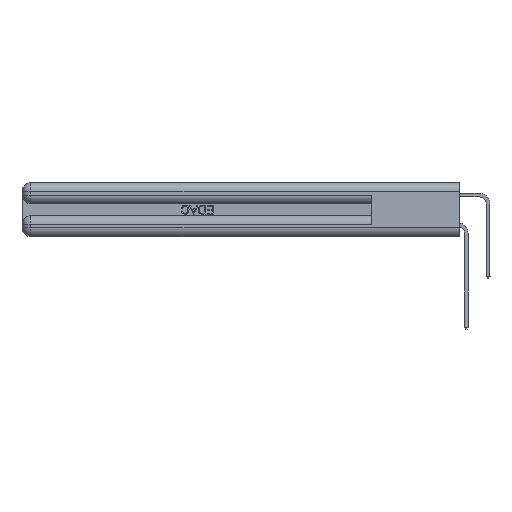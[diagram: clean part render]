
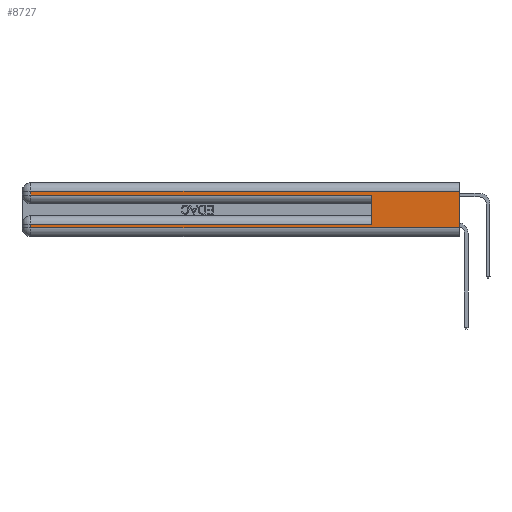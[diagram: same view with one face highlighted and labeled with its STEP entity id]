
A CAD part, left-side view. The second image highlights one B-rep face of the part: STEP entity #8727.
In plain terms, the highlighted planar face has unit normal (-1, 0, 0).
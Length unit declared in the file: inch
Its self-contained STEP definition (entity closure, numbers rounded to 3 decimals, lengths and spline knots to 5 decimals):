
#1024 = DIRECTION ( 'NONE',  ( 0., 0., -1. ) ) ;
#1883 = CARTESIAN_POINT ( 'NONE',  ( 0., 0., 0.31 ) ) ;
#2328 = EDGE_CURVE ( 'NONE', #23954, #23250, #42568, .T. ) ;
#2479 = EDGE_CURVE ( 'NONE', #31817, #32870, #14294, .T. ) ;
#4145 = VECTOR ( 'NONE', #5722, 39.37008 ) ;
#5465 = CARTESIAN_POINT ( 'NONE',  ( 0., 2.94, 0.31 ) ) ;
#5722 = DIRECTION ( 'NONE',  ( 0., 1., 0. ) ) ;
#5833 = VECTOR ( 'NONE', #11983, 39.37008 ) ;
#6729 = FACE_OUTER_BOUND ( 'NONE', #42413, .T. ) ;
#7518 = DIRECTION ( 'NONE',  ( 1., 0., 0. ) ) ;
#8128 = CARTESIAN_POINT ( 'NONE',  ( 0., 0.6, 0.145 ) ) ;
#8727 = ADVANCED_FACE ( 'NONE', ( #6729 ), #48818, .F. ) ;
#9153 = VERTEX_POINT ( 'NONE', #28420 ) ;
#10194 = VECTOR ( 'NONE', #19984, 39.37008 ) ;
#11245 = ORIENTED_EDGE ( 'NONE', *, *, #30647, .F. ) ;
#11983 = DIRECTION ( 'NONE',  ( 0., 0., 1. ) ) ;
#12028 = LINE ( 'NONE', #35225, #20831 ) ;
#12609 = DIRECTION ( 'NONE',  ( 0., -1., 0. ) ) ;
#14294 = LINE ( 'NONE', #1883, #4145 ) ;
#14537 = VECTOR ( 'NONE', #21253, 39.37008 ) ;
#14733 = CARTESIAN_POINT ( 'NONE',  ( 0., 0., 0.31 ) ) ;
#15948 = LINE ( 'NONE', #8128, #5833 ) ;
#17094 = CARTESIAN_POINT ( 'NONE',  ( 0., 0., 0.37 ) ) ;
#17153 = DIRECTION ( 'NONE',  ( 0., -1., 0. ) ) ;
#19131 = EDGE_CURVE ( 'NONE', #32870, #9153, #38466, .T. ) ;
#19954 = CARTESIAN_POINT ( 'NONE',  ( 0., 2.94, 0.37 ) ) ;
#19984 = DIRECTION ( 'NONE',  ( 0., 0., -1. ) ) ;
#20187 = CARTESIAN_POINT ( 'NONE',  ( 0., 0.6, 0.085 ) ) ;
#20487 = EDGE_CURVE ( 'NONE', #31817, #32474, #20671, .T. ) ;
#20541 = VERTEX_POINT ( 'NONE', #39964 ) ;
#20671 = LINE ( 'NONE', #17094, #29493 ) ;
#20831 = VECTOR ( 'NONE', #17153, 39.37008 ) ;
#21253 = DIRECTION ( 'NONE',  ( 0., 1., 0. ) ) ;
#21902 = ORIENTED_EDGE ( 'NONE', *, *, #34975, .T. ) ;
#23250 = VERTEX_POINT ( 'NONE', #28031 ) ;
#23479 = ORIENTED_EDGE ( 'NONE', *, *, #2328, .T. ) ;
#23733 = CARTESIAN_POINT ( 'NONE',  ( 0., 2.94, 0.37 ) ) ;
#23936 = ORIENTED_EDGE ( 'NONE', *, *, #34116, .T. ) ;
#23954 = VERTEX_POINT ( 'NONE', #28127 ) ;
#25112 = AXIS2_PLACEMENT_3D ( 'NONE', #33711, #7518, #33880 ) ;
#27268 = VECTOR ( 'NONE', #1024, 39.37008 ) ;
#27576 = CARTESIAN_POINT ( 'NONE',  ( 0., 0., 0.285 ) ) ;
#28031 = CARTESIAN_POINT ( 'NONE',  ( 0., 2.94, 0.06 ) ) ;
#28127 = CARTESIAN_POINT ( 'NONE',  ( 0., 2.94, 0.085 ) ) ;
#28420 = CARTESIAN_POINT ( 'NONE',  ( 0., 2.94, 0.285 ) ) ;
#29493 = VECTOR ( 'NONE', #47150, 39.37008 ) ;
#29786 = CARTESIAN_POINT ( 'NONE',  ( 0., 0., 0.06 ) ) ;
#30647 = EDGE_CURVE ( 'NONE', #44371, #20541, #15948, .T. ) ;
#31817 = VERTEX_POINT ( 'NONE', #14733 ) ;
#31900 = VECTOR ( 'NONE', #12609, 39.37008 ) ;
#32179 = ORIENTED_EDGE ( 'NONE', *, *, #41470, .T. ) ;
#32420 = CARTESIAN_POINT ( 'NONE',  ( 0., 0., 0.085 ) ) ;
#32474 = VERTEX_POINT ( 'NONE', #29786 ) ;
#32558 = ORIENTED_EDGE ( 'NONE', *, *, #2479, .T. ) ;
#32870 = VERTEX_POINT ( 'NONE', #5465 ) ;
#33711 = CARTESIAN_POINT ( 'NONE',  ( 0., 0., 0.37 ) ) ;
#33880 = DIRECTION ( 'NONE',  ( 0., 0., -1. ) ) ;
#34116 = EDGE_CURVE ( 'NONE', #23250, #32474, #12028, .T. ) ;
#34703 = ORIENTED_EDGE ( 'NONE', *, *, #19131, .T. ) ;
#34975 = EDGE_CURVE ( 'NONE', #9153, #20541, #35450, .T. ) ;
#34987 = ORIENTED_EDGE ( 'NONE', *, *, #20487, .F. ) ;
#35225 = CARTESIAN_POINT ( 'NONE',  ( 0., 0., 0.06 ) ) ;
#35450 = LINE ( 'NONE', #27576, #31900 ) ;
#38466 = LINE ( 'NONE', #19954, #27268 ) ;
#39964 = CARTESIAN_POINT ( 'NONE',  ( 0., 0.6, 0.285 ) ) ;
#41470 = EDGE_CURVE ( 'NONE', #44371, #23954, #44535, .T. ) ;
#42413 = EDGE_LOOP ( 'NONE', ( #34987, #32558, #34703, #21902, #11245, #32179, #23479, #23936 ) ) ;
#42568 = LINE ( 'NONE', #23733, #10194 ) ;
#44371 = VERTEX_POINT ( 'NONE', #20187 ) ;
#44535 = LINE ( 'NONE', #32420, #14537 ) ;
#47150 = DIRECTION ( 'NONE',  ( 0., 0., -1. ) ) ;
#48818 = PLANE ( 'NONE',  #25112 ) ;
